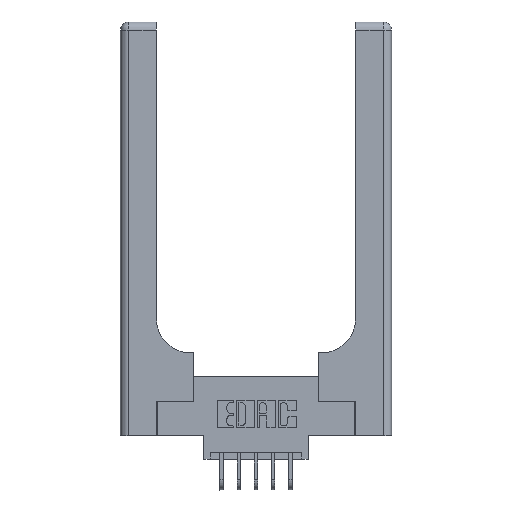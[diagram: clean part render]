
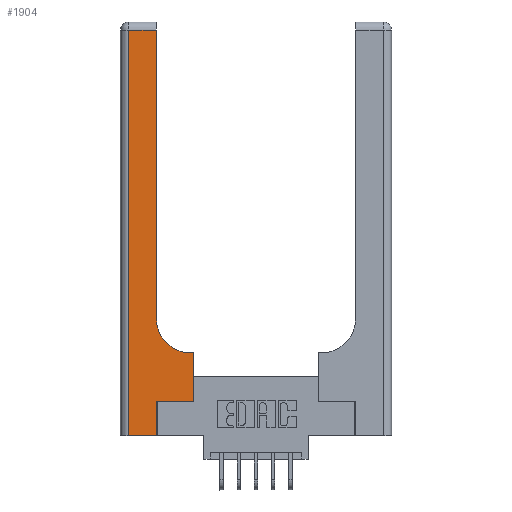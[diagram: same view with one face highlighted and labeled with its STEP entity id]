
A CAD part, top view. The second image highlights one B-rep face of the part: STEP entity #1904.
In plain terms, the highlighted planar face has unit normal (0, 0, 1).
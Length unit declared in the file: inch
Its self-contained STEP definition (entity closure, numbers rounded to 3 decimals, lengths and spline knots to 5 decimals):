
#55 = EDGE_CURVE ( 'NONE', #226, #6990, #2068, .T. ) ;
#69 = CARTESIAN_POINT ( 'NONE',  ( 0.06, 0., 0.37 ) ) ;
#226 = VERTEX_POINT ( 'NONE', #2101 ) ;
#248 = EDGE_CURVE ( 'NONE', #5942, #11587, #7224, .T. ) ;
#315 = DIRECTION ( 'NONE',  ( 0., 1., 0. ) ) ;
#516 = CARTESIAN_POINT ( 'NONE',  ( 0.528, 0.25, 0.37 ) ) ;
#668 = LINE ( 'NONE', #13704, #5673 ) ;
#672 = CIRCLE ( 'NONE', #12762, 0.25 ) ;
#718 = VERTEX_POINT ( 'NONE', #9564 ) ;
#776 = CARTESIAN_POINT ( 'NONE',  ( 0.06, 3., 0.37 ) ) ;
#1016 = EDGE_CURVE ( 'NONE', #11587, #226, #14628, .T. ) ;
#1278 = LINE ( 'NONE', #5801, #10933 ) ;
#1904 = ADVANCED_FACE ( 'NONE', ( #6165 ), #7583, .F. ) ;
#2068 = LINE ( 'NONE', #9009, #3921 ) ;
#2101 = CARTESIAN_POINT ( 'NONE',  ( 0.265, 0.25, 0.37 ) ) ;
#2306 = CARTESIAN_POINT ( 'NONE',  ( 0.26, 0.85, 0.37 ) ) ;
#2655 = VECTOR ( 'NONE', #4244, 39.37008 ) ;
#3783 = LINE ( 'NONE', #10254, #2655 ) ;
#3921 = VECTOR ( 'NONE', #12594, 39.37008 ) ;
#4217 = CARTESIAN_POINT ( 'NONE',  ( 0., 3., 0.37 ) ) ;
#4244 = DIRECTION ( 'NONE',  ( -1., 0., 0. ) ) ;
#4613 = DIRECTION ( 'NONE',  ( 0., -1., 0. ) ) ;
#4838 = DIRECTION ( 'NONE',  ( 0., 1., 0. ) ) ;
#4897 = VERTEX_POINT ( 'NONE', #2306 ) ;
#4950 = CARTESIAN_POINT ( 'NONE',  ( 0.265, 0., 0.37 ) ) ;
#5180 = ORIENTED_EDGE ( 'NONE', *, *, #6355, .T. ) ;
#5335 = EDGE_CURVE ( 'NONE', #718, #12197, #668, .T. ) ;
#5350 = LINE ( 'NONE', #10951, #10526 ) ;
#5673 = VECTOR ( 'NONE', #14723, 39.37008 ) ;
#5801 = CARTESIAN_POINT ( 'NONE',  ( 0.528, 0.25, 0.37 ) ) ;
#5817 = EDGE_CURVE ( 'NONE', #10774, #4897, #672, .T. ) ;
#5942 = VERTEX_POINT ( 'NONE', #69 ) ;
#5974 = CARTESIAN_POINT ( 'NONE',  ( 0.528, 0.6, 0.37 ) ) ;
#6165 = FACE_OUTER_BOUND ( 'NONE', #14747, .T. ) ;
#6355 = EDGE_CURVE ( 'NONE', #12197, #5942, #13662, .T. ) ;
#6639 = DIRECTION ( 'NONE',  ( 0., 0., -1. ) ) ;
#6851 = CARTESIAN_POINT ( 'NONE',  ( 0.51, 0.85, 0.37 ) ) ;
#6990 = VERTEX_POINT ( 'NONE', #516 ) ;
#7162 = VERTEX_POINT ( 'NONE', #5974 ) ;
#7202 = ORIENTED_EDGE ( 'NONE', *, *, #11437, .T. ) ;
#7224 = LINE ( 'NONE', #8122, #11143 ) ;
#7305 = EDGE_CURVE ( 'NONE', #7162, #10774, #3783, .T. ) ;
#7583 = PLANE ( 'NONE',  #11515 ) ;
#8122 = CARTESIAN_POINT ( 'NONE',  ( 0., 0., 0.37 ) ) ;
#8469 = ORIENTED_EDGE ( 'NONE', *, *, #248, .T. ) ;
#9009 = CARTESIAN_POINT ( 'NONE',  ( 0.265, 0.25, 0.37 ) ) ;
#9225 = CARTESIAN_POINT ( 'NONE',  ( 0.265, 0., 0.37 ) ) ;
#9257 = ORIENTED_EDGE ( 'NONE', *, *, #7305, .T. ) ;
#9323 = ORIENTED_EDGE ( 'NONE', *, *, #5817, .T. ) ;
#9564 = CARTESIAN_POINT ( 'NONE',  ( 0.26, 2.94, 0.37 ) ) ;
#9627 = ORIENTED_EDGE ( 'NONE', *, *, #5335, .T. ) ;
#9828 = ORIENTED_EDGE ( 'NONE', *, *, #15296, .T. ) ;
#9962 = CARTESIAN_POINT ( 'NONE',  ( 0.51, 0.6, 0.37 ) ) ;
#10249 = ORIENTED_EDGE ( 'NONE', *, *, #55, .T. ) ;
#10254 = CARTESIAN_POINT ( 'NONE',  ( 0.26, 0.6, 0.37 ) ) ;
#10526 = VECTOR ( 'NONE', #13236, 39.37008 ) ;
#10774 = VERTEX_POINT ( 'NONE', #9962 ) ;
#10933 = VECTOR ( 'NONE', #4838, 39.37008 ) ;
#10951 = CARTESIAN_POINT ( 'NONE',  ( 0.26, 3., 0.37 ) ) ;
#11105 = VECTOR ( 'NONE', #315, 39.37008 ) ;
#11143 = VECTOR ( 'NONE', #12828, 39.37008 ) ;
#11437 = EDGE_CURVE ( 'NONE', #4897, #718, #5350, .T. ) ;
#11515 = AXIS2_PLACEMENT_3D ( 'NONE', #4217, #6639, #13412 ) ;
#11587 = VERTEX_POINT ( 'NONE', #4950 ) ;
#11598 = DIRECTION ( 'NONE',  ( 1., 0., 0. ) ) ;
#12197 = VERTEX_POINT ( 'NONE', #15153 ) ;
#12594 = DIRECTION ( 'NONE',  ( 1., 0., 0. ) ) ;
#12758 = VECTOR ( 'NONE', #4613, 39.37008 ) ;
#12762 = AXIS2_PLACEMENT_3D ( 'NONE', #6851, #15193, #11598 ) ;
#12828 = DIRECTION ( 'NONE',  ( 1., 0., 0. ) ) ;
#13151 = ORIENTED_EDGE ( 'NONE', *, *, #1016, .T. ) ;
#13236 = DIRECTION ( 'NONE',  ( 0., 1., 0. ) ) ;
#13412 = DIRECTION ( 'NONE',  ( -1., 0., 0. ) ) ;
#13662 = LINE ( 'NONE', #776, #12758 ) ;
#13704 = CARTESIAN_POINT ( 'NONE',  ( 0., 2.94, 0.37 ) ) ;
#14628 = LINE ( 'NONE', #9225, #11105 ) ;
#14723 = DIRECTION ( 'NONE',  ( -1., 0., 0. ) ) ;
#14747 = EDGE_LOOP ( 'NONE', ( #7202, #9627, #5180, #8469, #13151, #10249, #9828, #9257, #9323 ) ) ;
#15153 = CARTESIAN_POINT ( 'NONE',  ( 0.06, 2.94, 0.37 ) ) ;
#15193 = DIRECTION ( 'NONE',  ( 0., 0., -1. ) ) ;
#15296 = EDGE_CURVE ( 'NONE', #6990, #7162, #1278, .T. ) ;
